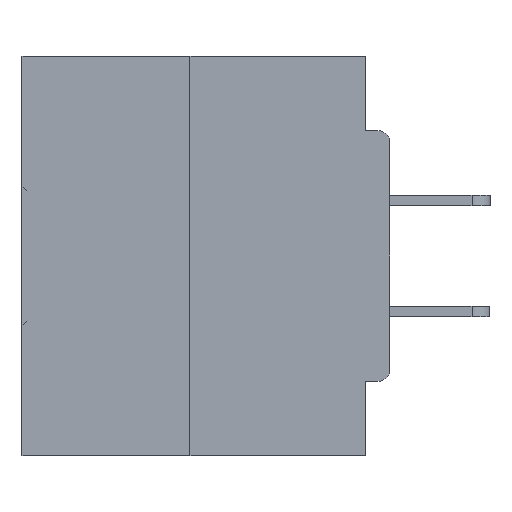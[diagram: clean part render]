
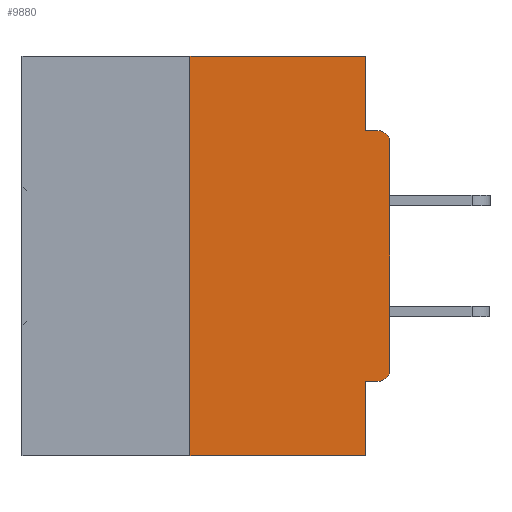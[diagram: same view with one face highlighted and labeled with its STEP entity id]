
A CAD part, left-side view. The second image highlights one B-rep face of the part: STEP entity #9880.
In plain terms, the highlighted planar face has unit normal (-1, 0, 0).
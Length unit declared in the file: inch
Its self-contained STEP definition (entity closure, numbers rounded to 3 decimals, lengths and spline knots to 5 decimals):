
#684 = VERTEX_POINT ( 'NONE', #21860 ) ;
#1126 = EDGE_CURVE ( 'NONE', #5554, #38425, #32908, .T. ) ;
#1350 = AXIS2_PLACEMENT_3D ( 'NONE', #15214, #35485, #1615 ) ;
#1422 = DIRECTION ( 'NONE',  ( -1., 0., 0. ) ) ;
#1615 = DIRECTION ( 'NONE',  ( 0., 0., -1. ) ) ;
#1662 = VERTEX_POINT ( 'NONE', #35765 ) ;
#2418 = VECTOR ( 'NONE', #12854, 39.37008 ) ;
#2864 = CARTESIAN_POINT ( 'NONE',  ( 0., 0.031, -0.4065 ) ) ;
#4138 = VECTOR ( 'NONE', #41211, 39.37008 ) ;
#5371 = PLANE ( 'NONE',  #30836 ) ;
#5424 = DIRECTION ( 'NONE',  ( 0., 0., 1. ) ) ;
#5554 = VERTEX_POINT ( 'NONE', #6289 ) ;
#5647 = DIRECTION ( 'NONE',  ( 1., 0., 0. ) ) ;
#5790 = DIRECTION ( 'NONE',  ( 0., 0., -1. ) ) ;
#5846 = VECTOR ( 'NONE', #26486, 39.37008 ) ;
#6001 = VECTOR ( 'NONE', #5424, 39.37008 ) ;
#6267 = AXIS2_PLACEMENT_3D ( 'NONE', #32028, #1422, #11752 ) ;
#6289 = CARTESIAN_POINT ( 'NONE',  ( 0., 0.031, -0.0935 ) ) ;
#6454 = ORIENTED_EDGE ( 'NONE', *, *, #39851, .F. ) ;
#6575 = LINE ( 'NONE', #9807, #19317 ) ;
#6828 = CARTESIAN_POINT ( 'NONE',  ( 0., 0., -0.4065 ) ) ;
#8576 = ORIENTED_EDGE ( 'NONE', *, *, #14932, .T. ) ;
#9164 = FACE_OUTER_BOUND ( 'NONE', #29213, .T. ) ;
#9807 = CARTESIAN_POINT ( 'NONE',  ( 0., 0.25, 0. ) ) ;
#9880 = ADVANCED_FACE ( 'NONE', ( #9164 ), #5371, .F. ) ;
#11752 = DIRECTION ( 'NONE',  ( 0., 0., -1. ) ) ;
#12854 = DIRECTION ( 'NONE',  ( 0., 0., -1. ) ) ;
#13095 = CARTESIAN_POINT ( 'NONE',  ( 0., 0.015, -0.0935 ) ) ;
#14101 = CARTESIAN_POINT ( 'NONE',  ( 0., 0., -0.0935 ) ) ;
#14911 = VERTEX_POINT ( 'NONE', #31028 ) ;
#14932 = EDGE_CURVE ( 'NONE', #25548, #38425, #20207, .T. ) ;
#15125 = EDGE_CURVE ( 'NONE', #14911, #684, #33420, .T. ) ;
#15214 = CARTESIAN_POINT ( 'NONE',  ( 0., 0.015, -0.1085 ) ) ;
#16593 = LINE ( 'NONE', #6828, #17155 ) ;
#17155 = VECTOR ( 'NONE', #30513, 39.37008 ) ;
#17555 = CARTESIAN_POINT ( 'NONE',  ( 0., 0.46, 0. ) ) ;
#18822 = CARTESIAN_POINT ( 'NONE',  ( 0., 0.46, 0. ) ) ;
#19146 = VERTEX_POINT ( 'NONE', #2864 ) ;
#19317 = VECTOR ( 'NONE', #21157, 39.37008 ) ;
#19562 = ORIENTED_EDGE ( 'NONE', *, *, #37749, .F. ) ;
#20207 = CIRCLE ( 'NONE', #1350, 0.015 ) ;
#21157 = DIRECTION ( 'NONE',  ( 0., 0., 1. ) ) ;
#21512 = EDGE_CURVE ( 'NONE', #21707, #1662, #33040, .T. ) ;
#21707 = VERTEX_POINT ( 'NONE', #22583 ) ;
#21828 = CARTESIAN_POINT ( 'NONE',  ( 0., 0., -0.1085 ) ) ;
#21833 = ORIENTED_EDGE ( 'NONE', *, *, #15125, .T. ) ;
#21860 = CARTESIAN_POINT ( 'NONE',  ( 0., 0.031, -0.5 ) ) ;
#22131 = CARTESIAN_POINT ( 'NONE',  ( 0., 0.031, 0. ) ) ;
#22583 = CARTESIAN_POINT ( 'NONE',  ( 0., 0.015, -0.4065 ) ) ;
#25548 = VERTEX_POINT ( 'NONE', #21828 ) ;
#26486 = DIRECTION ( 'NONE',  ( 0., 0., -1. ) ) ;
#28808 = ORIENTED_EDGE ( 'NONE', *, *, #1126, .F. ) ;
#29213 = EDGE_LOOP ( 'NONE', ( #19562, #37005, #21833, #43498, #6454, #40850, #33423, #8576, #28808, #43744 ) ) ;
#29467 = EDGE_CURVE ( 'NONE', #1662, #25548, #35669, .T. ) ;
#30149 = CARTESIAN_POINT ( 'NONE',  ( 0., 0.031, 0. ) ) ;
#30455 = LINE ( 'NONE', #30149, #2418 ) ;
#30513 = DIRECTION ( 'NONE',  ( 0., 1., 0. ) ) ;
#30836 = AXIS2_PLACEMENT_3D ( 'NONE', #18822, #5647, #5790 ) ;
#31028 = CARTESIAN_POINT ( 'NONE',  ( 0., 0.25, -0.5 ) ) ;
#31974 = EDGE_CURVE ( 'NONE', #19146, #684, #37108, .T. ) ;
#32028 = CARTESIAN_POINT ( 'NONE',  ( 0., 0.015, -0.3915 ) ) ;
#32484 = CARTESIAN_POINT ( 'NONE',  ( 0., 0., 0. ) ) ;
#32908 = LINE ( 'NONE', #14101, #39788 ) ;
#33040 = CIRCLE ( 'NONE', #6267, 0.015 ) ;
#33420 = LINE ( 'NONE', #36228, #41368 ) ;
#33423 = ORIENTED_EDGE ( 'NONE', *, *, #29467, .T. ) ;
#35379 = LINE ( 'NONE', #17555, #4138 ) ;
#35485 = DIRECTION ( 'NONE',  ( -1., 0., 0. ) ) ;
#35552 = VERTEX_POINT ( 'NONE', #40924 ) ;
#35669 = LINE ( 'NONE', #32484, #6001 ) ;
#35765 = CARTESIAN_POINT ( 'NONE',  ( 0., 0., -0.3915 ) ) ;
#36228 = CARTESIAN_POINT ( 'NONE',  ( 0., 0.46, -0.5 ) ) ;
#36436 = CARTESIAN_POINT ( 'NONE',  ( 0., 0.031, -0.5 ) ) ;
#37005 = ORIENTED_EDGE ( 'NONE', *, *, #39288, .F. ) ;
#37108 = LINE ( 'NONE', #36436, #5846 ) ;
#37337 = DIRECTION ( 'NONE',  ( 0., -1., 0. ) ) ;
#37749 = EDGE_CURVE ( 'NONE', #35552, #43510, #35379, .T. ) ;
#38425 = VERTEX_POINT ( 'NONE', #13095 ) ;
#39288 = EDGE_CURVE ( 'NONE', #14911, #35552, #6575, .T. ) ;
#39788 = VECTOR ( 'NONE', #37337, 39.37008 ) ;
#39851 = EDGE_CURVE ( 'NONE', #21707, #19146, #16593, .T. ) ;
#40850 = ORIENTED_EDGE ( 'NONE', *, *, #21512, .T. ) ;
#40924 = CARTESIAN_POINT ( 'NONE',  ( 0., 0.25, 0. ) ) ;
#41211 = DIRECTION ( 'NONE',  ( 0., -1., 0. ) ) ;
#41368 = VECTOR ( 'NONE', #42847, 39.37008 ) ;
#42847 = DIRECTION ( 'NONE',  ( 0., -1., 0. ) ) ;
#43498 = ORIENTED_EDGE ( 'NONE', *, *, #31974, .F. ) ;
#43510 = VERTEX_POINT ( 'NONE', #22131 ) ;
#43583 = EDGE_CURVE ( 'NONE', #43510, #5554, #30455, .T. ) ;
#43744 = ORIENTED_EDGE ( 'NONE', *, *, #43583, .F. ) ;
